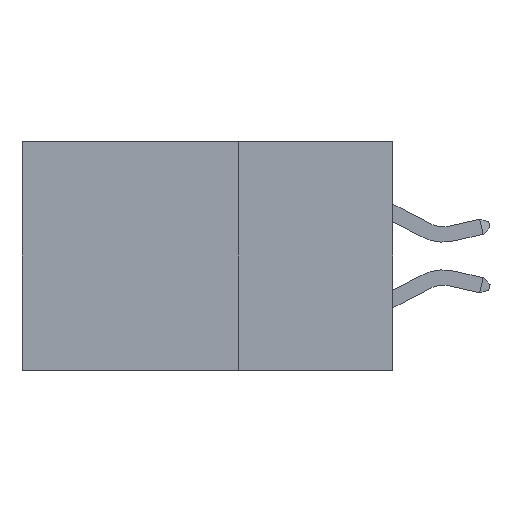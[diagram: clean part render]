
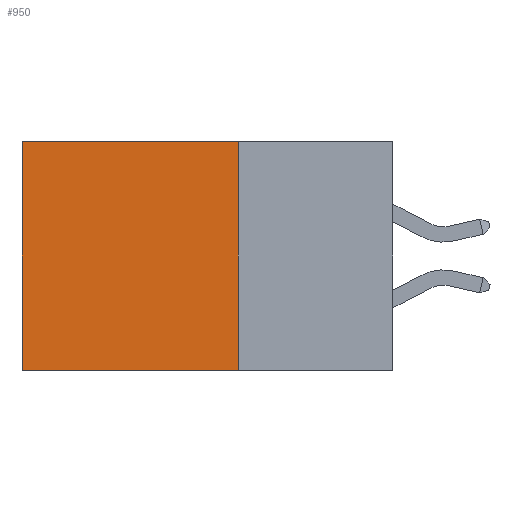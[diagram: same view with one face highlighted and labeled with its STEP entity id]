
A CAD part, left-side view. The second image highlights one B-rep face of the part: STEP entity #950.
In plain terms, the highlighted planar face has unit normal (-1, 0, 0).
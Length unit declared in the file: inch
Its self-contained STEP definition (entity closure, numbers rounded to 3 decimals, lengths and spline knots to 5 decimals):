
#303 = LINE ( 'NONE', #16141, #15890 ) ;
#950 = ADVANCED_FACE ( 'NONE', ( #12125 ), #7817, .F. ) ;
#966 = EDGE_CURVE ( 'NONE', #2835, #17248, #12594, .T. ) ;
#1755 = DIRECTION ( 'NONE',  ( 0., 0., -1. ) ) ;
#2728 = EDGE_LOOP ( 'NONE', ( #16516, #3624, #3741, #2791 ) ) ;
#2791 = ORIENTED_EDGE ( 'NONE', *, *, #966, .T. ) ;
#2835 = VERTEX_POINT ( 'NONE', #10744 ) ;
#3342 = CARTESIAN_POINT ( 'NONE',  ( 0.2875, 0.25, 0. ) ) ;
#3483 = CARTESIAN_POINT ( 'NONE',  ( 0.2875, 0.25, 0. ) ) ;
#3624 = ORIENTED_EDGE ( 'NONE', *, *, #4662, .F. ) ;
#3741 = ORIENTED_EDGE ( 'NONE', *, *, #4461, .F. ) ;
#3764 = LINE ( 'NONE', #15826, #11480 ) ;
#4461 = EDGE_CURVE ( 'NONE', #2835, #15474, #10771, .T. ) ;
#4662 = EDGE_CURVE ( 'NONE', #15474, #9836, #3764, .T. ) ;
#4793 = DIRECTION ( 'NONE',  ( 0., 1., 0. ) ) ;
#5153 = CARTESIAN_POINT ( 'NONE',  ( 0.2875, 0.25, 0. ) ) ;
#5169 = CARTESIAN_POINT ( 'NONE',  ( 0.2875, 0.6, 0. ) ) ;
#6844 = VECTOR ( 'NONE', #12587, 39.37008 ) ;
#7426 = AXIS2_PLACEMENT_3D ( 'NONE', #3342, #10737, #1755 ) ;
#7817 = PLANE ( 'NONE',  #7426 ) ;
#8615 = VECTOR ( 'NONE', #4793, 39.37008 ) ;
#9836 = VERTEX_POINT ( 'NONE', #11739 ) ;
#10737 = DIRECTION ( 'NONE',  ( 1., 0., 0. ) ) ;
#10744 = CARTESIAN_POINT ( 'NONE',  ( 0.2875, 0.25, 0. ) ) ;
#10771 = LINE ( 'NONE', #5153, #6844 ) ;
#11480 = VECTOR ( 'NONE', #11790, 39.37008 ) ;
#11739 = CARTESIAN_POINT ( 'NONE',  ( 0.2875, 0.6, -0.37 ) ) ;
#11790 = DIRECTION ( 'NONE',  ( 0., 1., 0. ) ) ;
#12125 = FACE_OUTER_BOUND ( 'NONE', #2728, .T. ) ;
#12587 = DIRECTION ( 'NONE',  ( 0., 0., -1. ) ) ;
#12594 = LINE ( 'NONE', #3483, #8615 ) ;
#15474 = VERTEX_POINT ( 'NONE', #15962 ) ;
#15826 = CARTESIAN_POINT ( 'NONE',  ( 0.2875, 0.25, -0.37 ) ) ;
#15890 = VECTOR ( 'NONE', #16080, 39.37008 ) ;
#15962 = CARTESIAN_POINT ( 'NONE',  ( 0.2875, 0.25, -0.37 ) ) ;
#16080 = DIRECTION ( 'NONE',  ( 0., 0., -1. ) ) ;
#16141 = CARTESIAN_POINT ( 'NONE',  ( 0.2875, 0.6, 0. ) ) ;
#16516 = ORIENTED_EDGE ( 'NONE', *, *, #17575, .T. ) ;
#17248 = VERTEX_POINT ( 'NONE', #5169 ) ;
#17575 = EDGE_CURVE ( 'NONE', #17248, #9836, #303, .T. ) ;
